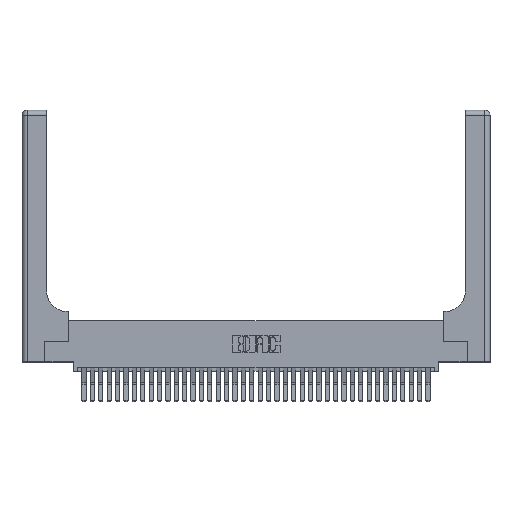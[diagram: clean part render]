
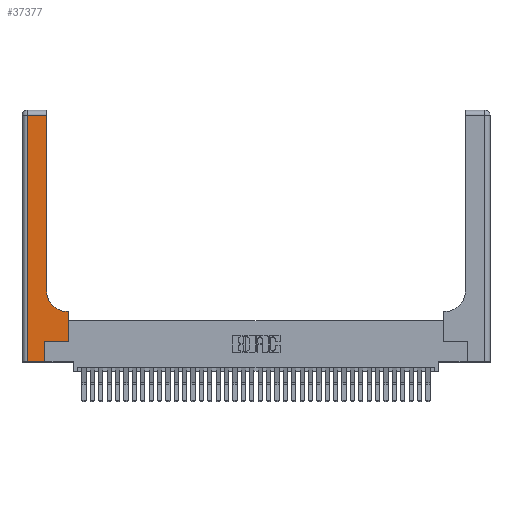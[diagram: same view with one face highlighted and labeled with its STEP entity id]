
A CAD part, top view. The second image highlights one B-rep face of the part: STEP entity #37377.
In plain terms, the highlighted planar face has unit normal (0, 0, 1).
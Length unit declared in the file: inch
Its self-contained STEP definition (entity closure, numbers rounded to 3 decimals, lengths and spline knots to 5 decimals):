
#446 = EDGE_CURVE ( 'NONE', #12189, #37462, #32134, .T. ) ;
#1197 = CARTESIAN_POINT ( 'NONE',  ( 0.269, 0., 0.37 ) ) ;
#2635 = ORIENTED_EDGE ( 'NONE', *, *, #15806, .T. ) ;
#3001 = FACE_OUTER_BOUND ( 'NONE', #30049, .T. ) ;
#3179 = VERTEX_POINT ( 'NONE', #26080 ) ;
#3775 = VECTOR ( 'NONE', #23967, 39.37008 ) ;
#4791 = DIRECTION ( 'NONE',  ( 0., 0., -1. ) ) ;
#5384 = LINE ( 'NONE', #6514, #24863 ) ;
#5393 = VERTEX_POINT ( 'NONE', #17726 ) ;
#5648 = CARTESIAN_POINT ( 'NONE',  ( 0.2915, 0.6, 0.37 ) ) ;
#6031 = CARTESIAN_POINT ( 'NONE',  ( 0., 0., 0.37 ) ) ;
#6163 = DIRECTION ( 'NONE',  ( 1., 0., 0. ) ) ;
#6514 = CARTESIAN_POINT ( 'NONE',  ( 0., 2.94, 0.37 ) ) ;
#6547 = LINE ( 'NONE', #32727, #3775 ) ;
#6870 = VECTOR ( 'NONE', #25250, 39.37008 ) ;
#8067 = EDGE_CURVE ( 'NONE', #32812, #15092, #37606, .T. ) ;
#9517 = EDGE_CURVE ( 'NONE', #32180, #5393, #34508, .T. ) ;
#11230 = AXIS2_PLACEMENT_3D ( 'NONE', #35703, #26807, #6163 ) ;
#11254 = CARTESIAN_POINT ( 'NONE',  ( 0.06, 0., 0.37 ) ) ;
#12189 = VERTEX_POINT ( 'NONE', #29302 ) ;
#12323 = VECTOR ( 'NONE', #23741, 39.37008 ) ;
#12777 = CARTESIAN_POINT ( 'NONE',  ( 0.06, 3., 0.37 ) ) ;
#13566 = DIRECTION ( 'NONE',  ( 1., 0., 0. ) ) ;
#13949 = EDGE_CURVE ( 'NONE', #15092, #20468, #33679, .T. ) ;
#14049 = ORIENTED_EDGE ( 'NONE', *, *, #446, .T. ) ;
#14957 = DIRECTION ( 'NONE',  ( -1., 0., 0. ) ) ;
#15092 = VERTEX_POINT ( 'NONE', #23592 ) ;
#15107 = CARTESIAN_POINT ( 'NONE',  ( 0.5585, 0.6, 0.37 ) ) ;
#15806 = EDGE_CURVE ( 'NONE', #26784, #32812, #6547, .T. ) ;
#15938 = CARTESIAN_POINT ( 'NONE',  ( 0.5585, 0.25, 0.37 ) ) ;
#16249 = VECTOR ( 'NONE', #32360, 39.37008 ) ;
#17272 = EDGE_CURVE ( 'NONE', #20468, #3179, #23683, .T. ) ;
#17726 = CARTESIAN_POINT ( 'NONE',  ( 0.269, 0.25, 0.37 ) ) ;
#19318 = ORIENTED_EDGE ( 'NONE', *, *, #28496, .T. ) ;
#19826 = ORIENTED_EDGE ( 'NONE', *, *, #28750, .T. ) ;
#20302 = LINE ( 'NONE', #6031, #12323 ) ;
#20468 = VERTEX_POINT ( 'NONE', #37445 ) ;
#21296 = CARTESIAN_POINT ( 'NONE',  ( 0.269, 0., 0.37 ) ) ;
#21665 = ORIENTED_EDGE ( 'NONE', *, *, #9517, .T. ) ;
#22462 = ORIENTED_EDGE ( 'NONE', *, *, #13949, .T. ) ;
#23592 = CARTESIAN_POINT ( 'NONE',  ( 0.5415, 0.6, 0.37 ) ) ;
#23683 = LINE ( 'NONE', #29551, #6870 ) ;
#23741 = DIRECTION ( 'NONE',  ( 1., 0., 0. ) ) ;
#23967 = DIRECTION ( 'NONE',  ( 0., 1., 0. ) ) ;
#24863 = VECTOR ( 'NONE', #14957, 39.37008 ) ;
#25250 = DIRECTION ( 'NONE',  ( 0., 1., 0. ) ) ;
#25590 = PLANE ( 'NONE',  #31641 ) ;
#26060 = ORIENTED_EDGE ( 'NONE', *, *, #8067, .T. ) ;
#26080 = CARTESIAN_POINT ( 'NONE',  ( 0.2915, 2.94, 0.37 ) ) ;
#26784 = VERTEX_POINT ( 'NONE', #15938 ) ;
#26807 = DIRECTION ( 'NONE',  ( 0., 0., -1. ) ) ;
#27903 = DIRECTION ( 'NONE',  ( 0., 1., 0. ) ) ;
#28407 = DIRECTION ( 'NONE',  ( -1., 0., 0. ) ) ;
#28496 = EDGE_CURVE ( 'NONE', #3179, #12189, #5384, .T. ) ;
#28582 = LINE ( 'NONE', #37270, #30401 ) ;
#28750 = EDGE_CURVE ( 'NONE', #5393, #26784, #28582, .T. ) ;
#29302 = CARTESIAN_POINT ( 'NONE',  ( 0.06, 2.94, 0.37 ) ) ;
#29551 = CARTESIAN_POINT ( 'NONE',  ( 0.2915, 3., 0.37 ) ) ;
#29887 = ORIENTED_EDGE ( 'NONE', *, *, #17272, .T. ) ;
#30049 = EDGE_LOOP ( 'NONE', ( #29887, #19318, #14049, #36952, #21665, #19826, #2635, #26060, #22462 ) ) ;
#30401 = VECTOR ( 'NONE', #13566, 39.37008 ) ;
#30764 = VECTOR ( 'NONE', #36493, 39.37008 ) ;
#31641 = AXIS2_PLACEMENT_3D ( 'NONE', #34206, #4791, #28407 ) ;
#32134 = LINE ( 'NONE', #12777, #30764 ) ;
#32180 = VERTEX_POINT ( 'NONE', #21296 ) ;
#32360 = DIRECTION ( 'NONE',  ( -1., 0., 0. ) ) ;
#32727 = CARTESIAN_POINT ( 'NONE',  ( 0.5585, 0.25, 0.37 ) ) ;
#32812 = VERTEX_POINT ( 'NONE', #15107 ) ;
#33558 = VECTOR ( 'NONE', #27903, 39.37008 ) ;
#33679 = CIRCLE ( 'NONE', #11230, 0.25 ) ;
#34206 = CARTESIAN_POINT ( 'NONE',  ( 0., 3., 0.37 ) ) ;
#34508 = LINE ( 'NONE', #1197, #33558 ) ;
#35703 = CARTESIAN_POINT ( 'NONE',  ( 0.5415, 0.85, 0.37 ) ) ;
#36257 = EDGE_CURVE ( 'NONE', #37462, #32180, #20302, .T. ) ;
#36493 = DIRECTION ( 'NONE',  ( 0., -1., 0. ) ) ;
#36952 = ORIENTED_EDGE ( 'NONE', *, *, #36257, .T. ) ;
#37270 = CARTESIAN_POINT ( 'NONE',  ( 0.269, 0.25, 0.37 ) ) ;
#37377 = ADVANCED_FACE ( 'NONE', ( #3001 ), #25590, .F. ) ;
#37445 = CARTESIAN_POINT ( 'NONE',  ( 0.2915, 0.85, 0.37 ) ) ;
#37462 = VERTEX_POINT ( 'NONE', #11254 ) ;
#37606 = LINE ( 'NONE', #5648, #16249 ) ;
